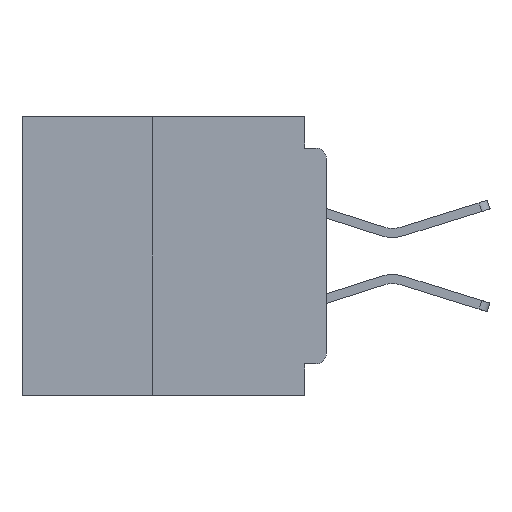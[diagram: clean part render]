
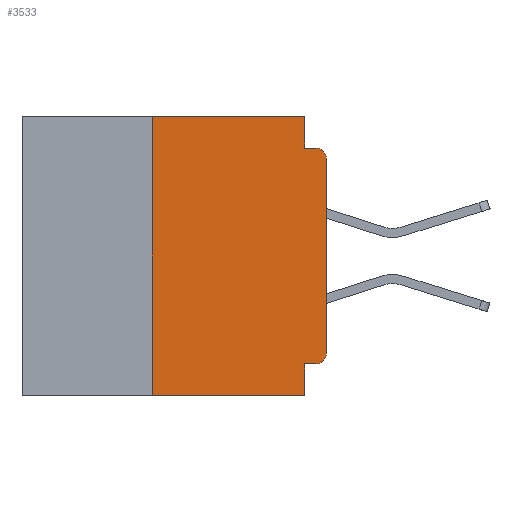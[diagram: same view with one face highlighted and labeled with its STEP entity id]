
A CAD part, left-side view. The second image highlights one B-rep face of the part: STEP entity #3533.
In plain terms, the highlighted planar face has unit normal (-1, 0, 0).
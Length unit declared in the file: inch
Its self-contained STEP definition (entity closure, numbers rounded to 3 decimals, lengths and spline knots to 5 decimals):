
#203 = CIRCLE ( 'NONE', #16861, 0.015 ) ;
#510 = VECTOR ( 'NONE', #22435, 39.37008 ) ;
#632 = DIRECTION ( 'NONE',  ( 0., 0., -1. ) ) ;
#1425 = ORIENTED_EDGE ( 'NONE', *, *, #16732, .F. ) ;
#1434 = LINE ( 'NONE', #24050, #9220 ) ;
#1821 = CARTESIAN_POINT ( 'NONE',  ( 0., 0.031, -0.045 ) ) ;
#2407 = LINE ( 'NONE', #35581, #18995 ) ;
#2563 = LINE ( 'NONE', #40503, #10380 ) ;
#2578 = LINE ( 'NONE', #28920, #510 ) ;
#3533 = ADVANCED_FACE ( 'NONE', ( #25889 ), #36904, .F. ) ;
#3990 = ORIENTED_EDGE ( 'NONE', *, *, #22956, .T. ) ;
#4181 = EDGE_CURVE ( 'NONE', #10041, #19377, #25081, .T. ) ;
#5036 = EDGE_CURVE ( 'NONE', #16622, #29689, #203, .T. ) ;
#5681 = DIRECTION ( 'NONE',  ( -1., 0., 0. ) ) ;
#5834 = CARTESIAN_POINT ( 'NONE',  ( 0., 0.031, -0.355 ) ) ;
#6677 = LINE ( 'NONE', #41845, #34118 ) ;
#7159 = EDGE_CURVE ( 'NONE', #16622, #39767, #41360, .T. ) ;
#7308 = EDGE_LOOP ( 'NONE', ( #38113, #3990, #30407, #41201, #24731, #1425, #12329, #38652, #13356, #15861 ) ) ;
#9220 = VECTOR ( 'NONE', #10905, 39.37008 ) ;
#10041 = VERTEX_POINT ( 'NONE', #10616 ) ;
#10380 = VECTOR ( 'NONE', #20764, 39.37008 ) ;
#10616 = CARTESIAN_POINT ( 'NONE',  ( 0., 0.031, 0. ) ) ;
#10905 = DIRECTION ( 'NONE',  ( 0., 0., 1. ) ) ;
#11113 = CARTESIAN_POINT ( 'NONE',  ( 0., 0.031, -0.4 ) ) ;
#12221 = VERTEX_POINT ( 'NONE', #40505 ) ;
#12329 = ORIENTED_EDGE ( 'NONE', *, *, #14911, .T. ) ;
#12827 = CARTESIAN_POINT ( 'NONE',  ( 0., 0.25, -0.4 ) ) ;
#13356 = ORIENTED_EDGE ( 'NONE', *, *, #7159, .F. ) ;
#14911 = EDGE_CURVE ( 'NONE', #33478, #37913, #2578, .T. ) ;
#15861 = ORIENTED_EDGE ( 'NONE', *, *, #5036, .T. ) ;
#16622 = VERTEX_POINT ( 'NONE', #26924 ) ;
#16732 = EDGE_CURVE ( 'NONE', #33478, #12221, #1434, .T. ) ;
#16752 = CARTESIAN_POINT ( 'NONE',  ( 0., 0.015, -0.045 ) ) ;
#16861 = AXIS2_PLACEMENT_3D ( 'NONE', #25511, #5681, #28824 ) ;
#17142 = CARTESIAN_POINT ( 'NONE',  ( 0., 0.437, 0. ) ) ;
#17960 = CARTESIAN_POINT ( 'NONE',  ( 0., 0.015, -0.06 ) ) ;
#18814 = DIRECTION ( 'NONE',  ( 0., -1., 0. ) ) ;
#18995 = VECTOR ( 'NONE', #42152, 39.37008 ) ;
#19377 = VERTEX_POINT ( 'NONE', #1821 ) ;
#19573 = VERTEX_POINT ( 'NONE', #16752 ) ;
#20463 = DIRECTION ( 'NONE',  ( 1., 0., 0. ) ) ;
#20764 = DIRECTION ( 'NONE',  ( 0., 0., 1. ) ) ;
#20924 = DIRECTION ( 'NONE',  ( 0., 0., -1. ) ) ;
#21280 = DIRECTION ( 'NONE',  ( 0., 0., -1. ) ) ;
#22151 = EDGE_CURVE ( 'NONE', #29689, #28494, #2563, .T. ) ;
#22435 = DIRECTION ( 'NONE',  ( 0., -1., 0. ) ) ;
#22956 = EDGE_CURVE ( 'NONE', #28494, #19573, #41313, .T. ) ;
#23128 = EDGE_CURVE ( 'NONE', #12221, #10041, #6677, .T. ) ;
#23918 = DIRECTION ( 'NONE',  ( 0., 1., 0. ) ) ;
#24050 = CARTESIAN_POINT ( 'NONE',  ( 0., 0.25, -0.4 ) ) ;
#24063 = VECTOR ( 'NONE', #27490, 39.37008 ) ;
#24158 = CARTESIAN_POINT ( 'NONE',  ( 0., 0., -0.34 ) ) ;
#24543 = LINE ( 'NONE', #11113, #32292 ) ;
#24580 = EDGE_CURVE ( 'NONE', #19377, #19573, #2407, .T. ) ;
#24731 = ORIENTED_EDGE ( 'NONE', *, *, #23128, .F. ) ;
#25081 = LINE ( 'NONE', #37296, #24063 ) ;
#25511 = CARTESIAN_POINT ( 'NONE',  ( 0., 0.015, -0.34 ) ) ;
#25889 = FACE_OUTER_BOUND ( 'NONE', #7308, .T. ) ;
#26924 = CARTESIAN_POINT ( 'NONE',  ( 0., 0.015, -0.355 ) ) ;
#27220 = CARTESIAN_POINT ( 'NONE',  ( 0., 0., -0.355 ) ) ;
#27490 = DIRECTION ( 'NONE',  ( 0., 0., -1. ) ) ;
#28494 = VERTEX_POINT ( 'NONE', #36642 ) ;
#28824 = DIRECTION ( 'NONE',  ( 0., 0., -1. ) ) ;
#28920 = CARTESIAN_POINT ( 'NONE',  ( 0., 0.437, -0.4 ) ) ;
#29586 = AXIS2_PLACEMENT_3D ( 'NONE', #17960, #41015, #21280 ) ;
#29689 = VERTEX_POINT ( 'NONE', #24158 ) ;
#30407 = ORIENTED_EDGE ( 'NONE', *, *, #24580, .F. ) ;
#32292 = VECTOR ( 'NONE', #20924, 39.37008 ) ;
#33478 = VERTEX_POINT ( 'NONE', #12827 ) ;
#34118 = VECTOR ( 'NONE', #18814, 39.37008 ) ;
#35581 = CARTESIAN_POINT ( 'NONE',  ( 0., 0., -0.045 ) ) ;
#36642 = CARTESIAN_POINT ( 'NONE',  ( 0., 0., -0.06 ) ) ;
#36904 = PLANE ( 'NONE',  #38668 ) ;
#37296 = CARTESIAN_POINT ( 'NONE',  ( 0., 0.031, 0. ) ) ;
#37913 = VERTEX_POINT ( 'NONE', #40995 ) ;
#38113 = ORIENTED_EDGE ( 'NONE', *, *, #22151, .T. ) ;
#38280 = VECTOR ( 'NONE', #23918, 39.37008 ) ;
#38485 = EDGE_CURVE ( 'NONE', #39767, #37913, #24543, .T. ) ;
#38652 = ORIENTED_EDGE ( 'NONE', *, *, #38485, .F. ) ;
#38668 = AXIS2_PLACEMENT_3D ( 'NONE', #17142, #20463, #632 ) ;
#39767 = VERTEX_POINT ( 'NONE', #5834 ) ;
#40503 = CARTESIAN_POINT ( 'NONE',  ( 0., 0., 0. ) ) ;
#40505 = CARTESIAN_POINT ( 'NONE',  ( 0., 0.25, 0. ) ) ;
#40995 = CARTESIAN_POINT ( 'NONE',  ( 0., 0.031, -0.4 ) ) ;
#41015 = DIRECTION ( 'NONE',  ( -1., 0., 0. ) ) ;
#41201 = ORIENTED_EDGE ( 'NONE', *, *, #4181, .F. ) ;
#41313 = CIRCLE ( 'NONE', #29586, 0.015 ) ;
#41360 = LINE ( 'NONE', #27220, #38280 ) ;
#41845 = CARTESIAN_POINT ( 'NONE',  ( 0., 0.437, 0. ) ) ;
#42152 = DIRECTION ( 'NONE',  ( 0., -1., 0. ) ) ;
